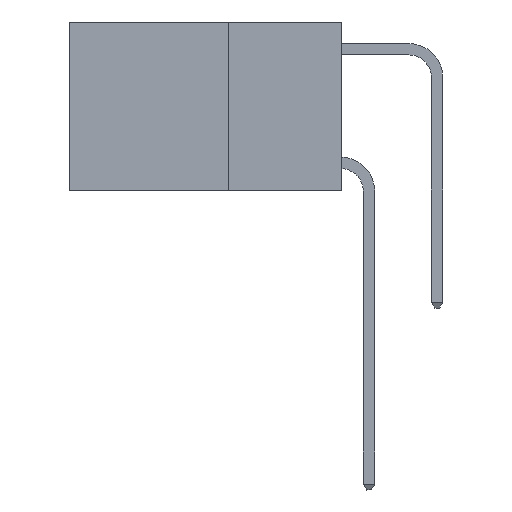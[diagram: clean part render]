
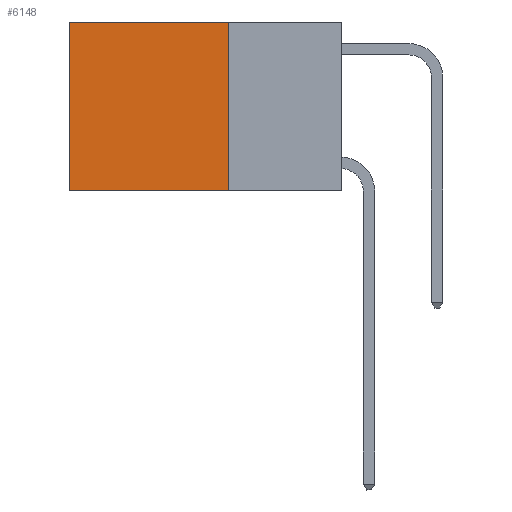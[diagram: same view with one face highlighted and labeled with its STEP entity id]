
A CAD part, left-side view. The second image highlights one B-rep face of the part: STEP entity #6148.
In plain terms, the highlighted planar face has unit normal (-1, 0, 0).
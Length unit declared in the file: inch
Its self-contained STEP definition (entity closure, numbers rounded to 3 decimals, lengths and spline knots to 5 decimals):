
#52 = DIRECTION ( 'NONE',  ( 0., 1., 0. ) ) ;
#84 = EDGE_CURVE ( 'NONE', #11428, #12559, #2985, .T. ) ;
#773 = VERTEX_POINT ( 'NONE', #10372 ) ;
#829 = VECTOR ( 'NONE', #4537, 39.37008 ) ;
#876 = DIRECTION ( 'NONE',  ( 0., 1., 0. ) ) ;
#1081 = LINE ( 'NONE', #11769, #8660 ) ;
#1699 = CARTESIAN_POINT ( 'NONE',  ( 0.2625, 0.25, 0. ) ) ;
#1747 = LINE ( 'NONE', #2792, #4395 ) ;
#2077 = VERTEX_POINT ( 'NONE', #4933 ) ;
#2473 = ORIENTED_EDGE ( 'NONE', *, *, #7509, .F. ) ;
#2792 = CARTESIAN_POINT ( 'NONE',  ( 0.2625, 0.6, 0. ) ) ;
#2985 = LINE ( 'NONE', #4763, #10806 ) ;
#3742 = PLANE ( 'NONE',  #10043 ) ;
#4395 = VECTOR ( 'NONE', #12481, 39.37008 ) ;
#4402 = CARTESIAN_POINT ( 'NONE',  ( 0.2625, 0.6, 0. ) ) ;
#4537 = DIRECTION ( 'NONE',  ( 0., 0., -1. ) ) ;
#4734 = DIRECTION ( 'NONE',  ( 0., 0., -1. ) ) ;
#4763 = CARTESIAN_POINT ( 'NONE',  ( 0.2625, 0.25, 0. ) ) ;
#4933 = CARTESIAN_POINT ( 'NONE',  ( 0.2625, 0.25, -0.37 ) ) ;
#5364 = EDGE_LOOP ( 'NONE', ( #8544, #5529, #2473, #8720 ) ) ;
#5529 = ORIENTED_EDGE ( 'NONE', *, *, #10786, .F. ) ;
#6148 = ADVANCED_FACE ( 'NONE', ( #8589 ), #3742, .F. ) ;
#7509 = EDGE_CURVE ( 'NONE', #11428, #2077, #10396, .T. ) ;
#8379 = EDGE_CURVE ( 'NONE', #12559, #773, #1747, .T. ) ;
#8544 = ORIENTED_EDGE ( 'NONE', *, *, #8379, .T. ) ;
#8589 = FACE_OUTER_BOUND ( 'NONE', #5364, .T. ) ;
#8660 = VECTOR ( 'NONE', #52, 39.37008 ) ;
#8720 = ORIENTED_EDGE ( 'NONE', *, *, #84, .T. ) ;
#10043 = AXIS2_PLACEMENT_3D ( 'NONE', #1699, #10596, #4734 ) ;
#10372 = CARTESIAN_POINT ( 'NONE',  ( 0.2625, 0.6, -0.37 ) ) ;
#10396 = LINE ( 'NONE', #11344, #829 ) ;
#10596 = DIRECTION ( 'NONE',  ( 1., 0., 0. ) ) ;
#10683 = CARTESIAN_POINT ( 'NONE',  ( 0.2625, 0.25, 0. ) ) ;
#10786 = EDGE_CURVE ( 'NONE', #2077, #773, #1081, .T. ) ;
#10806 = VECTOR ( 'NONE', #876, 39.37008 ) ;
#11344 = CARTESIAN_POINT ( 'NONE',  ( 0.2625, 0.25, 0. ) ) ;
#11428 = VERTEX_POINT ( 'NONE', #10683 ) ;
#11769 = CARTESIAN_POINT ( 'NONE',  ( 0.2625, 0.25, -0.37 ) ) ;
#12481 = DIRECTION ( 'NONE',  ( 0., 0., -1. ) ) ;
#12559 = VERTEX_POINT ( 'NONE', #4402 ) ;
